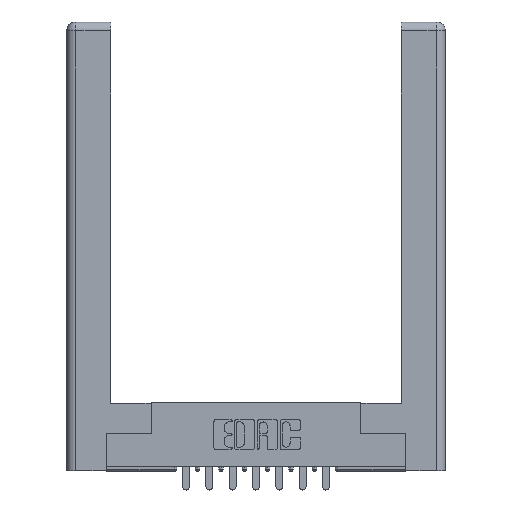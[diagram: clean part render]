
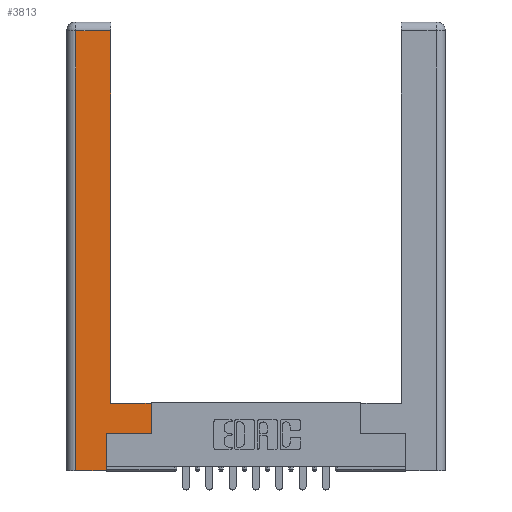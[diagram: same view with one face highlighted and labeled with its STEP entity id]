
A CAD part, top view. The second image highlights one B-rep face of the part: STEP entity #3813.
In plain terms, the highlighted planar face has unit normal (0, 0, 1).
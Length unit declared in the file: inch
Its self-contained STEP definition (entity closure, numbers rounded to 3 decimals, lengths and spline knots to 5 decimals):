
#168 = EDGE_CURVE ( 'NONE', #10203, #13336, #12286, .T. ) ;
#253 = EDGE_CURVE ( 'NONE', #2402, #2672, #3442, .T. ) ;
#402 = VERTEX_POINT ( 'NONE', #8089 ) ;
#732 = VECTOR ( 'NONE', #6099, 39.37008 ) ;
#896 = CARTESIAN_POINT ( 'NONE',  ( 0.0615, 2.94, 0. ) ) ;
#943 = DIRECTION ( 'NONE',  ( 0., -1., 0. ) ) ;
#1000 = CARTESIAN_POINT ( 'NONE',  ( 0.265, 0., 0. ) ) ;
#1035 = CARTESIAN_POINT ( 'NONE',  ( 0.295, 3., 0. ) ) ;
#1182 = ORIENTED_EDGE ( 'NONE', *, *, #168, .T. ) ;
#1477 = EDGE_CURVE ( 'NONE', #13336, #9948, #7187, .T. ) ;
#1835 = VECTOR ( 'NONE', #9784, 39.37008 ) ;
#1949 = EDGE_CURVE ( 'NONE', #2672, #10203, #10838, .T. ) ;
#1961 = DIRECTION ( 'NONE',  ( -1., 0., 0. ) ) ;
#2047 = VECTOR ( 'NONE', #3236, 39.37008 ) ;
#2350 = CARTESIAN_POINT ( 'NONE',  ( 0.295, 2.94, 0. ) ) ;
#2402 = VERTEX_POINT ( 'NONE', #6624 ) ;
#2581 = DIRECTION ( 'NONE',  ( 1., 0., 0. ) ) ;
#2672 = VERTEX_POINT ( 'NONE', #6821 ) ;
#2689 = EDGE_CURVE ( 'NONE', #402, #5642, #12741, .T. ) ;
#3236 = DIRECTION ( 'NONE',  ( -1., 0., 0. ) ) ;
#3442 = LINE ( 'NONE', #9915, #7596 ) ;
#3577 = EDGE_CURVE ( 'NONE', #5642, #2402, #11491, .T. ) ;
#3813 = ADVANCED_FACE ( 'NONE', ( #7680 ), #4210, .F. ) ;
#4163 = DIRECTION ( 'NONE',  ( 0., 0., -1. ) ) ;
#4210 = PLANE ( 'NONE',  #7587 ) ;
#4549 = VERTEX_POINT ( 'NONE', #6950 ) ;
#4796 = LINE ( 'NONE', #896, #1835 ) ;
#4934 = CARTESIAN_POINT ( 'NONE',  ( 0.265, 0., 0. ) ) ;
#5275 = VECTOR ( 'NONE', #8249, 39.37008 ) ;
#5461 = CARTESIAN_POINT ( 'NONE',  ( 0.0615, 0., 0. ) ) ;
#5642 = VERTEX_POINT ( 'NONE', #1000 ) ;
#6047 = DIRECTION ( 'NONE',  ( 0., 1., 0. ) ) ;
#6099 = DIRECTION ( 'NONE',  ( 0., 1., 0. ) ) ;
#6143 = CARTESIAN_POINT ( 'NONE',  ( 0.565, 0.45, 0. ) ) ;
#6624 = CARTESIAN_POINT ( 'NONE',  ( 0.265, 0.245, 0. ) ) ;
#6686 = EDGE_CURVE ( 'NONE', #4549, #402, #9197, .T. ) ;
#6821 = CARTESIAN_POINT ( 'NONE',  ( 0.565, 0.245, 0. ) ) ;
#6950 = CARTESIAN_POINT ( 'NONE',  ( 0.0615, 2.94, 0. ) ) ;
#7187 = LINE ( 'NONE', #1035, #8590 ) ;
#7298 = ORIENTED_EDGE ( 'NONE', *, *, #2689, .T. ) ;
#7587 = AXIS2_PLACEMENT_3D ( 'NONE', #11947, #4163, #1961 ) ;
#7596 = VECTOR ( 'NONE', #2581, 39.37008 ) ;
#7680 = FACE_OUTER_BOUND ( 'NONE', #12146, .T. ) ;
#8089 = CARTESIAN_POINT ( 'NONE',  ( 0.0615, 0., 0. ) ) ;
#8219 = VECTOR ( 'NONE', #6047, 39.37008 ) ;
#8249 = DIRECTION ( 'NONE',  ( 1., 0., 0. ) ) ;
#8369 = ORIENTED_EDGE ( 'NONE', *, *, #1949, .T. ) ;
#8590 = VECTOR ( 'NONE', #9728, 39.37008 ) ;
#9157 = ORIENTED_EDGE ( 'NONE', *, *, #6686, .T. ) ;
#9197 = LINE ( 'NONE', #5461, #13018 ) ;
#9615 = CARTESIAN_POINT ( 'NONE',  ( 0.565, 0.45, 0. ) ) ;
#9698 = EDGE_CURVE ( 'NONE', #9948, #4549, #4796, .T. ) ;
#9728 = DIRECTION ( 'NONE',  ( 0., 1., 0. ) ) ;
#9784 = DIRECTION ( 'NONE',  ( -1., 0., 0. ) ) ;
#9915 = CARTESIAN_POINT ( 'NONE',  ( 0.565, 0.245, 0. ) ) ;
#9948 = VERTEX_POINT ( 'NONE', #2350 ) ;
#9968 = CARTESIAN_POINT ( 'NONE',  ( 0.295, 0.45, 0. ) ) ;
#10203 = VERTEX_POINT ( 'NONE', #9615 ) ;
#10557 = ORIENTED_EDGE ( 'NONE', *, *, #3577, .T. ) ;
#10838 = LINE ( 'NONE', #6143, #8219 ) ;
#11491 = LINE ( 'NONE', #12772, #732 ) ;
#11947 = CARTESIAN_POINT ( 'NONE',  ( 0., 0., 0. ) ) ;
#12146 = EDGE_LOOP ( 'NONE', ( #12331, #12702, #9157, #7298, #10557, #14045, #8369, #1182 ) ) ;
#12286 = LINE ( 'NONE', #13882, #2047 ) ;
#12331 = ORIENTED_EDGE ( 'NONE', *, *, #1477, .T. ) ;
#12702 = ORIENTED_EDGE ( 'NONE', *, *, #9698, .T. ) ;
#12741 = LINE ( 'NONE', #4934, #5275 ) ;
#12772 = CARTESIAN_POINT ( 'NONE',  ( 0.265, 0.245, 0. ) ) ;
#13018 = VECTOR ( 'NONE', #943, 39.37008 ) ;
#13336 = VERTEX_POINT ( 'NONE', #9968 ) ;
#13882 = CARTESIAN_POINT ( 'NONE',  ( 0.295, 0.45, 0. ) ) ;
#14045 = ORIENTED_EDGE ( 'NONE', *, *, #253, .T. ) ;
